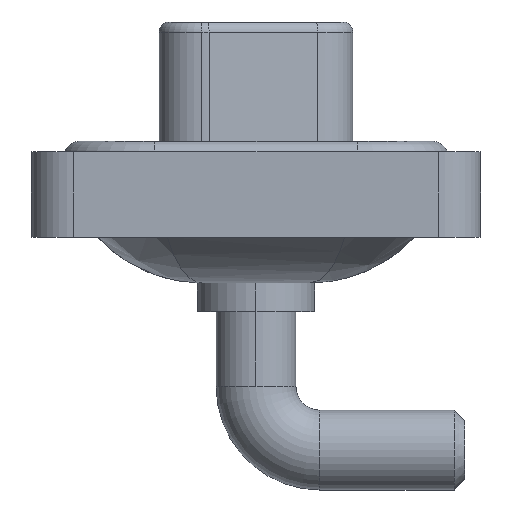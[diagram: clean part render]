
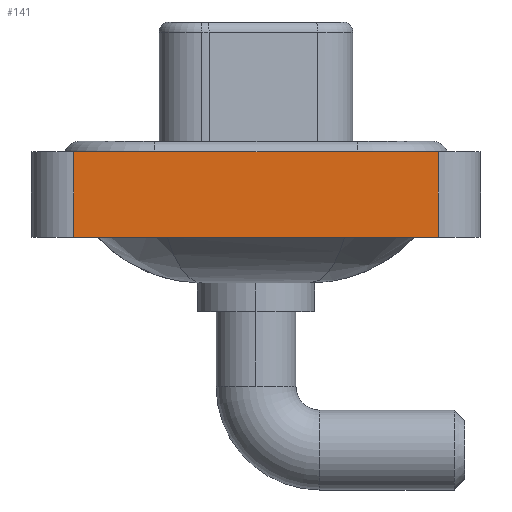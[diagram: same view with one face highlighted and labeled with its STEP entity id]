
A CAD part, left-side view. The second image highlights one B-rep face of the part: STEP entity #141.
In plain terms, the highlighted planar face has unit normal (-1, 0, 0).
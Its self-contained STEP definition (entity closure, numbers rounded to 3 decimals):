
#141 = ADVANCED_FACE ( 'NONE', ( #619 ), #10905, .T. ) ;
#376 = CARTESIAN_POINT ( 'NONE',  ( -7.25, -8.55, -3.6 ) ) ;
#619 = FACE_OUTER_BOUND ( 'NONE', #3970, .T. ) ;
#842 = ORIENTED_EDGE ( 'NONE', *, *, #13441, .F. ) ;
#1120 = LINE ( 'NONE', #3233, #1181 ) ;
#1150 = VECTOR ( 'NONE', #2943, 1000. ) ;
#1181 = VECTOR ( 'NONE', #7876, 1000. ) ;
#1825 = DIRECTION ( 'NONE',  ( 0., -1., 0. ) ) ;
#1900 = EDGE_CURVE ( 'NONE', #8086, #4725, #14642, .T. ) ;
#1967 = VECTOR ( 'NONE', #1825, 1000. ) ;
#2791 = CARTESIAN_POINT ( 'NONE',  ( -7.25, 8.55, -3.6 ) ) ;
#2943 = DIRECTION ( 'NONE',  ( 0., -1., 0. ) ) ;
#3219 = VECTOR ( 'NONE', #6479, 1000. ) ;
#3233 = CARTESIAN_POINT ( 'NONE',  ( -7.25, 8.55, -3.6 ) ) ;
#3729 = CARTESIAN_POINT ( 'NONE',  ( -7.25, 8.55, 0.4 ) ) ;
#3970 = EDGE_LOOP ( 'NONE', ( #9130, #11437, #842, #4614 ) ) ;
#4347 = CARTESIAN_POINT ( 'NONE',  ( -7.25, -8.55, -3.6 ) ) ;
#4614 = ORIENTED_EDGE ( 'NONE', *, *, #7218, .T. ) ;
#4725 = VERTEX_POINT ( 'NONE', #5789 ) ;
#5242 = DIRECTION ( 'NONE',  ( 0., 0., 1. ) ) ;
#5789 = CARTESIAN_POINT ( 'NONE',  ( -7.25, -8.55, 0.4 ) ) ;
#6296 = LINE ( 'NONE', #376, #1150 ) ;
#6479 = DIRECTION ( 'NONE',  ( 0., 0., 1. ) ) ;
#6553 = EDGE_CURVE ( 'NONE', #12592, #4725, #12275, .T. ) ;
#7218 = EDGE_CURVE ( 'NONE', #13232, #8086, #6296, .T. ) ;
#7876 = DIRECTION ( 'NONE',  ( 0., 0., 1. ) ) ;
#8086 = VERTEX_POINT ( 'NONE', #4347 ) ;
#9130 = ORIENTED_EDGE ( 'NONE', *, *, #1900, .T. ) ;
#9449 = AXIS2_PLACEMENT_3D ( 'NONE', #12119, #13126, #5242 ) ;
#10905 = PLANE ( 'NONE',  #9449 ) ;
#10910 = CARTESIAN_POINT ( 'NONE',  ( -7.25, -8.55, 0.4 ) ) ;
#11437 = ORIENTED_EDGE ( 'NONE', *, *, #6553, .F. ) ;
#12119 = CARTESIAN_POINT ( 'NONE',  ( -7.25, -8.55, -3.6 ) ) ;
#12222 = CARTESIAN_POINT ( 'NONE',  ( -7.25, -8.55, -3.6 ) ) ;
#12275 = LINE ( 'NONE', #10910, #1967 ) ;
#12592 = VERTEX_POINT ( 'NONE', #3729 ) ;
#13126 = DIRECTION ( 'NONE',  ( -1., 0., 0. ) ) ;
#13232 = VERTEX_POINT ( 'NONE', #2791 ) ;
#13441 = EDGE_CURVE ( 'NONE', #13232, #12592, #1120, .T. ) ;
#14642 = LINE ( 'NONE', #12222, #3219 ) ;
